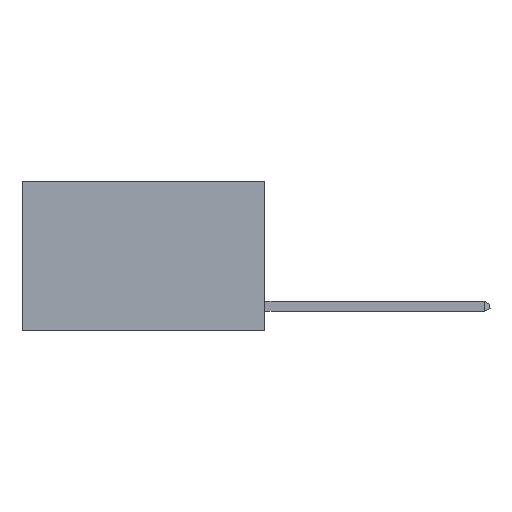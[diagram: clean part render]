
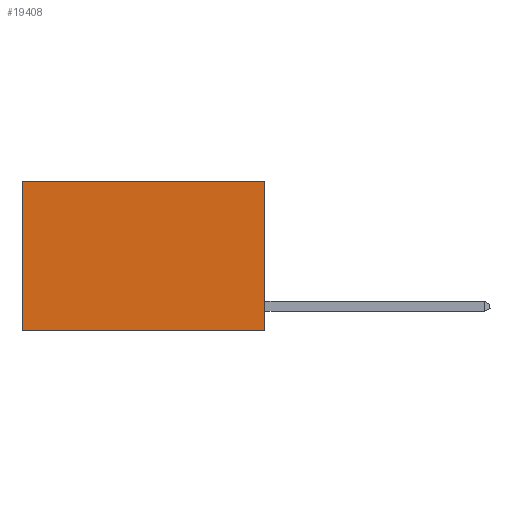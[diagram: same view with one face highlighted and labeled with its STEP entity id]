
A CAD part, left-side view. The second image highlights one B-rep face of the part: STEP entity #19408.
In plain terms, the highlighted planar face has unit normal (-1, 0, 0).
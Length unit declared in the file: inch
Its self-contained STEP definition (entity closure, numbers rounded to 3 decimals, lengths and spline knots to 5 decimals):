
#58 = CARTESIAN_POINT ( 'NONE',  ( 0.2625, 0., 0. ) ) ;
#1879 = CARTESIAN_POINT ( 'NONE',  ( 0.2625, 0., 0. ) ) ;
#2144 = DIRECTION ( 'NONE',  ( 0., 0., -1. ) ) ;
#4344 = EDGE_CURVE ( 'NONE', #17475, #9232, #24343, .T. ) ;
#5021 = DIRECTION ( 'NONE',  ( 0., 1., 0. ) ) ;
#8458 = CARTESIAN_POINT ( 'NONE',  ( 0.2625, 0., 0. ) ) ;
#8884 = EDGE_CURVE ( 'NONE', #25680, #9232, #14151, .T. ) ;
#8973 = CARTESIAN_POINT ( 'NONE',  ( 0.2625, 0.6, 0. ) ) ;
#9232 = VERTEX_POINT ( 'NONE', #24098 ) ;
#9600 = VECTOR ( 'NONE', #27159, 39.37008 ) ;
#10758 = DIRECTION ( 'NONE',  ( 0., 0., -1. ) ) ;
#11003 = ORIENTED_EDGE ( 'NONE', *, *, #4344, .F. ) ;
#13613 = CARTESIAN_POINT ( 'NONE',  ( 0.2625, 0.6, 0. ) ) ;
#13948 = EDGE_CURVE ( 'NONE', #21862, #17475, #27814, .T. ) ;
#14151 = LINE ( 'NONE', #13613, #25619 ) ;
#15268 = PLANE ( 'NONE',  #17422 ) ;
#15296 = ORIENTED_EDGE ( 'NONE', *, *, #8884, .T. ) ;
#16162 = EDGE_LOOP ( 'NONE', ( #15296, #11003, #27188, #20576 ) ) ;
#17422 = AXIS2_PLACEMENT_3D ( 'NONE', #8458, #24452, #10758 ) ;
#17475 = VERTEX_POINT ( 'NONE', #22202 ) ;
#18750 = CARTESIAN_POINT ( 'NONE',  ( 0.2625, 0., -0.37 ) ) ;
#19408 = ADVANCED_FACE ( 'NONE', ( #27979 ), #15268, .F. ) ;
#19657 = EDGE_CURVE ( 'NONE', #21862, #25680, #26878, .T. ) ;
#20576 = ORIENTED_EDGE ( 'NONE', *, *, #19657, .T. ) ;
#20742 = DIRECTION ( 'NONE',  ( 0., 1., 0. ) ) ;
#20812 = VECTOR ( 'NONE', #20742, 39.37008 ) ;
#21862 = VERTEX_POINT ( 'NONE', #1879 ) ;
#22202 = CARTESIAN_POINT ( 'NONE',  ( 0.2625, 0., -0.37 ) ) ;
#24098 = CARTESIAN_POINT ( 'NONE',  ( 0.2625, 0.6, -0.37 ) ) ;
#24343 = LINE ( 'NONE', #18750, #29692 ) ;
#24452 = DIRECTION ( 'NONE',  ( 1., 0., 0. ) ) ;
#24871 = CARTESIAN_POINT ( 'NONE',  ( 0.2625, 0., 0. ) ) ;
#25619 = VECTOR ( 'NONE', #2144, 39.37008 ) ;
#25680 = VERTEX_POINT ( 'NONE', #8973 ) ;
#26878 = LINE ( 'NONE', #58, #20812 ) ;
#27159 = DIRECTION ( 'NONE',  ( 0., 0., -1. ) ) ;
#27188 = ORIENTED_EDGE ( 'NONE', *, *, #13948, .F. ) ;
#27814 = LINE ( 'NONE', #24871, #9600 ) ;
#27979 = FACE_OUTER_BOUND ( 'NONE', #16162, .T. ) ;
#29692 = VECTOR ( 'NONE', #5021, 39.37008 ) ;
